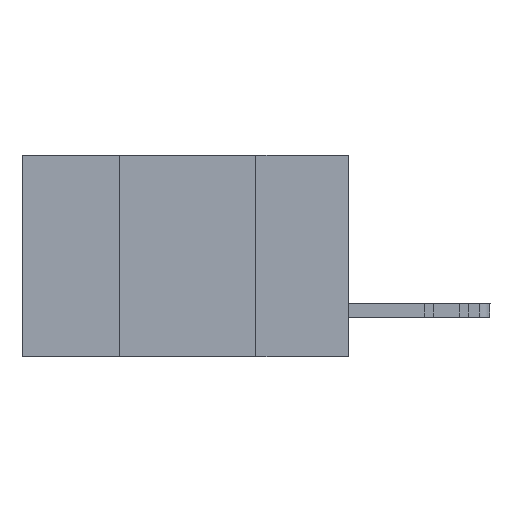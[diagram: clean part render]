
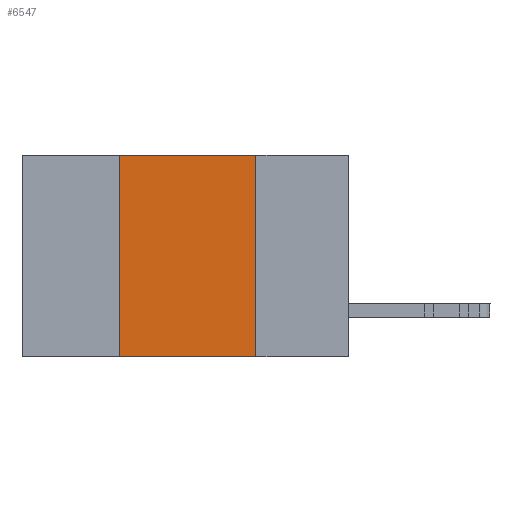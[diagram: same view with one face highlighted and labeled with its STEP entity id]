
A CAD part, left-side view. The second image highlights one B-rep face of the part: STEP entity #6547.
In plain terms, the highlighted planar face has unit normal (-1, 0, 0).
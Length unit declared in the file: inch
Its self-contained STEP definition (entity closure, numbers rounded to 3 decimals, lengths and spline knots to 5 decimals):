
#1658 = VERTEX_POINT ( 'NONE', #24408 ) ;
#3313 = VECTOR ( 'NONE', #23191, 39.37008 ) ;
#3362 = ORIENTED_EDGE ( 'NONE', *, *, #21339, .T. ) ;
#3391 = EDGE_CURVE ( 'NONE', #14638, #1658, #3822, .T. ) ;
#3650 = FACE_OUTER_BOUND ( 'NONE', #4016, .T. ) ;
#3822 = LINE ( 'NONE', #13259, #13594 ) ;
#4016 = EDGE_LOOP ( 'NONE', ( #10469, #5223, #19954, #3362 ) ) ;
#5081 = VECTOR ( 'NONE', #8986, 39.37008 ) ;
#5082 = VERTEX_POINT ( 'NONE', #24511 ) ;
#5223 = ORIENTED_EDGE ( 'NONE', *, *, #3391, .F. ) ;
#6547 = ADVANCED_FACE ( 'NONE', ( #3650 ), #19280, .F. ) ;
#7128 = CARTESIAN_POINT ( 'NONE',  ( 0., 0.6, -0.37 ) ) ;
#7880 = EDGE_CURVE ( 'NONE', #1658, #20984, #19882, .T. ) ;
#8951 = CARTESIAN_POINT ( 'NONE',  ( 0., 0.42, 0. ) ) ;
#8986 = DIRECTION ( 'NONE',  ( 0., -1., 0. ) ) ;
#9033 = DIRECTION ( 'NONE',  ( 0., 0., -1. ) ) ;
#9906 = CARTESIAN_POINT ( 'NONE',  ( 0., 0.17, -0.37 ) ) ;
#10231 = LINE ( 'NONE', #7128, #5081 ) ;
#10469 = ORIENTED_EDGE ( 'NONE', *, *, #7880, .F. ) ;
#13259 = CARTESIAN_POINT ( 'NONE',  ( 0., 0.6, 0. ) ) ;
#13339 = DIRECTION ( 'NONE',  ( 0., -1., 0. ) ) ;
#13594 = VECTOR ( 'NONE', #13339, 39.37008 ) ;
#14353 = VECTOR ( 'NONE', #9033, 39.37008 ) ;
#14638 = VERTEX_POINT ( 'NONE', #8951 ) ;
#16916 = CARTESIAN_POINT ( 'NONE',  ( 0., 0.17, -0.37 ) ) ;
#18411 = DIRECTION ( 'NONE',  ( 0., 0., -1. ) ) ;
#18415 = DIRECTION ( 'NONE',  ( 1., 0., 0. ) ) ;
#18677 = LINE ( 'NONE', #21362, #3313 ) ;
#19077 = CARTESIAN_POINT ( 'NONE',  ( 0., 0.6, 0. ) ) ;
#19280 = PLANE ( 'NONE',  #20793 ) ;
#19882 = LINE ( 'NONE', #16916, #14353 ) ;
#19954 = ORIENTED_EDGE ( 'NONE', *, *, #24510, .F. ) ;
#20793 = AXIS2_PLACEMENT_3D ( 'NONE', #19077, #18415, #18411 ) ;
#20984 = VERTEX_POINT ( 'NONE', #9906 ) ;
#21339 = EDGE_CURVE ( 'NONE', #5082, #20984, #10231, .T. ) ;
#21362 = CARTESIAN_POINT ( 'NONE',  ( 0., 0.42, -0.37 ) ) ;
#23191 = DIRECTION ( 'NONE',  ( 0., 0., 1. ) ) ;
#24408 = CARTESIAN_POINT ( 'NONE',  ( 0., 0.17, 0. ) ) ;
#24510 = EDGE_CURVE ( 'NONE', #5082, #14638, #18677, .T. ) ;
#24511 = CARTESIAN_POINT ( 'NONE',  ( 0., 0.42, -0.37 ) ) ;
